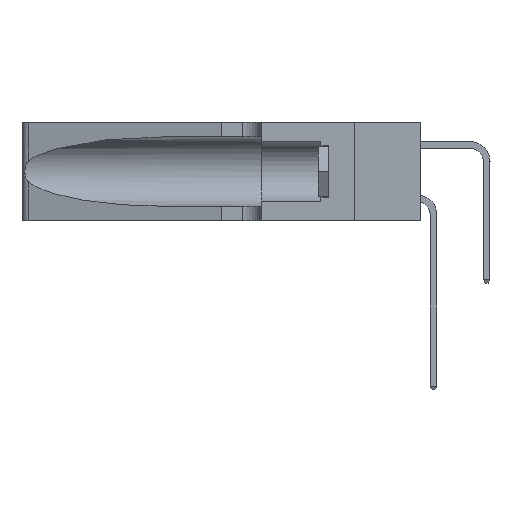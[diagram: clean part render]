
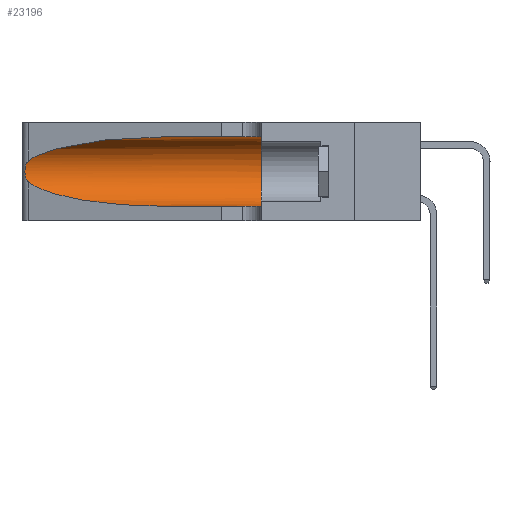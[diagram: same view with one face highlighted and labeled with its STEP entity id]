
A CAD part, left-side view. The second image highlights one B-rep face of the part: STEP entity #23196.
In plain terms, the highlighted cylindrical face has radius 3.308 mm (diameter 6.617 mm), a partial arc.
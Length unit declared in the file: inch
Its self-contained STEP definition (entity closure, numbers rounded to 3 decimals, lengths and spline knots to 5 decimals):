
#501 = CARTESIAN_POINT ( 'NONE',  ( 0.1305, 0.35, 0.31525 ) ) ;
#938 = CIRCLE ( 'NONE', #2635, 0.13025 ) ;
#1178 = AXIS2_PLACEMENT_3D ( 'NONE', #28094, #37419, #25106 ) ;
#1410 = CARTESIAN_POINT ( 'NONE',  ( 0.25487, 1.22718, 0.22369 ) ) ;
#1908 = CARTESIAN_POINT ( 'NONE',  ( 0.26018, 1.23835, 0.19895 ) ) ;
#2635 = AXIS2_PLACEMENT_3D ( 'NONE', #4890, #23425, #38960 ) ;
#3471 = CARTESIAN_POINT ( 'NONE',  ( 0.1305, 0.72297, 0.05475 ) ) ;
#3901 = VERTEX_POINT ( 'NONE', #39192 ) ;
#4736 = CARTESIAN_POINT ( 'NONE',  ( 0.25787, 1.23484, 0.2124 ) ) ;
#4890 = CARTESIAN_POINT ( 'NONE',  ( 0.1305, 0.35, 0.185 ) ) ;
#5528 = CARTESIAN_POINT ( 'NONE',  ( 0.25555, 1.22993, 0.14849 ) ) ;
#6198 = VERTEX_POINT ( 'NONE', #37043 ) ;
#7622 = CARTESIAN_POINT ( 'NONE',  ( 0.1305, 0.72297, 0.31525 ) ) ;
#8643 = ORIENTED_EDGE ( 'NONE', *, *, #38091, .T. ) ;
#9295 = CARTESIAN_POINT ( 'NONE',  ( 0.25487, 1.22718, 0.14631 ) ) ;
#9516 =( BOUNDED_CURVE ( )  B_SPLINE_CURVE ( 3, ( #13980, #20180, #32379, #16548 ),
 .UNSPECIFIED., .F., .T. ) 
 B_SPLINE_CURVE_WITH_KNOTS ( ( 4, 4 ),
 ( 1.5708, 2.84003 ),
 .UNSPECIFIED. ) 
 CURVE ( )  GEOMETRIC_REPRESENTATION_ITEM ( )  RATIONAL_B_SPLINE_CURVE ( ( 1., 0.87, 0.87, 1. ) ) 
 REPRESENTATION_ITEM ( '' )  );
#10037 = EDGE_CURVE ( 'NONE', #26850, #33340, #9516, .T. ) ;
#10630 = DIRECTION ( 'NONE',  ( 0., -1., 0. ) ) ;
#10841 = CARTESIAN_POINT ( 'NONE',  ( 0.25555, 1.22994, 0.2215 ) ) ;
#12903 = CYLINDRICAL_SURFACE ( 'NONE', #1178, 0.13025 ) ;
#13160 = LINE ( 'NONE', #38216, #28650 ) ;
#13615 = EDGE_CURVE ( 'NONE', #33340, #6198, #37051, .T. ) ;
#13980 = CARTESIAN_POINT ( 'NONE',  ( 0.1305, 0.72297, 0.31525 ) ) ;
#14177 = CARTESIAN_POINT ( 'NONE',  ( 0.25639, 1.23184, 0.21858 ) ) ;
#14317 = CARTESIAN_POINT ( 'NONE',  ( 0.26075, 1.23896, 0.19203 ) ) ;
#15771 = CARTESIAN_POINT ( 'NONE',  ( 0.18966, 0.96281, 0.05475 ) ) ;
#16548 = CARTESIAN_POINT ( 'NONE',  ( 0.25487, 1.22718, 0.22369 ) ) ;
#17108 = EDGE_CURVE ( 'NONE', #26850, #18586, #21584, .T. ) ;
#17307 = CARTESIAN_POINT ( 'NONE',  ( 0.26075, 1.23896, 0.178 ) ) ;
#17739 = ORIENTED_EDGE ( 'NONE', *, *, #13615, .T. ) ;
#18586 = VERTEX_POINT ( 'NONE', #501 ) ;
#18624 = CARTESIAN_POINT ( 'NONE',  ( 0.2373, 1.15595, 0.08982 ) ) ;
#19341 = ORIENTED_EDGE ( 'NONE', *, *, #17108, .F. ) ;
#20180 = CARTESIAN_POINT ( 'NONE',  ( 0.18966, 0.96281, 0.31525 ) ) ;
#20257 = CARTESIAN_POINT ( 'NONE',  ( 0.25487, 1.22718, 0.22369 ) ) ;
#21584 = LINE ( 'NONE', #36576, #24023 ) ;
#23081 = EDGE_LOOP ( 'NONE', ( #36023, #17739, #30147, #8643, #28327, #19341 ) ) ;
#23196 = ADVANCED_FACE ( 'NONE', ( #26982 ), #12903, .F. ) ;
#23425 = DIRECTION ( 'NONE',  ( 0., 1., 0. ) ) ;
#23883 = DIRECTION ( 'NONE',  ( 0., -1., 0. ) ) ;
#24023 = VECTOR ( 'NONE', #23883, 39.37008 ) ;
#25106 = DIRECTION ( 'NONE',  ( 0., 0., -1. ) ) ;
#26850 = VERTEX_POINT ( 'NONE', #7622 ) ;
#26982 = FACE_OUTER_BOUND ( 'NONE', #23081, .T. ) ;
#27190 = CARTESIAN_POINT ( 'NONE',  ( 0.25487, 1.22718, 0.14631 ) ) ;
#28094 = CARTESIAN_POINT ( 'NONE',  ( 0.1305, 1.61858, 0.185 ) ) ;
#28327 = ORIENTED_EDGE ( 'NONE', *, *, #32774, .F. ) ;
#28650 = VECTOR ( 'NONE', #10630, 39.37008 ) ;
#29889 = CARTESIAN_POINT ( 'NONE',  ( 0.25639, 1.23186, 0.15144 ) ) ;
#30147 = ORIENTED_EDGE ( 'NONE', *, *, #30730, .T. ) ;
#30158 = CARTESIAN_POINT ( 'NONE',  ( 0.25789, 1.23486, 0.15765 ) ) ;
#30730 = EDGE_CURVE ( 'NONE', #6198, #37258, #39515, .T. ) ;
#32379 = CARTESIAN_POINT ( 'NONE',  ( 0.2373, 1.15595, 0.28018 ) ) ;
#32774 = EDGE_CURVE ( 'NONE', #18586, #3901, #938, .T. ) ;
#32981 = CARTESIAN_POINT ( 'NONE',  ( 0.1305, 0.72297, 0.05475 ) ) ;
#33340 = VERTEX_POINT ( 'NONE', #1410 ) ;
#36023 = ORIENTED_EDGE ( 'NONE', *, *, #10037, .T. ) ;
#36576 = CARTESIAN_POINT ( 'NONE',  ( 0.1305, 1.61858, 0.31525 ) ) ;
#37043 = CARTESIAN_POINT ( 'NONE',  ( 0.25487, 1.22718, 0.14631 ) ) ;
#37051 = B_SPLINE_CURVE_WITH_KNOTS ( 'NONE', 3,
 ( #20257, #10841, #14177, #4736, #38285, #1908, #14317, #17307, #38931, #39195, #30158, #29889, #5528, #27190 ),
 .UNSPECIFIED., .F., .F.,
 ( 4, 2, 2, 2, 2, 2, 4 ),
 ( 0., 0.00027, 0.00053, 0.00107, 0.0016, 0.00187, 0.00214 ),
 .UNSPECIFIED. ) ;
#37258 = VERTEX_POINT ( 'NONE', #32981 ) ;
#37419 = DIRECTION ( 'NONE',  ( 0., -1., 0. ) ) ;
#38091 = EDGE_CURVE ( 'NONE', #37258, #3901, #13160, .T. ) ;
#38216 = CARTESIAN_POINT ( 'NONE',  ( 0.1305, 1.61858, 0.05475 ) ) ;
#38285 = CARTESIAN_POINT ( 'NONE',  ( 0.25854, 1.2359, 0.20912 ) ) ;
#38931 = CARTESIAN_POINT ( 'NONE',  ( 0.26017, 1.23833, 0.17102 ) ) ;
#38960 = DIRECTION ( 'NONE',  ( 0., 0., 1. ) ) ;
#39192 = CARTESIAN_POINT ( 'NONE',  ( 0.1305, 0.35, 0.05475 ) ) ;
#39195 = CARTESIAN_POINT ( 'NONE',  ( 0.25856, 1.23593, 0.16098 ) ) ;
#39515 =( BOUNDED_CURVE ( )  B_SPLINE_CURVE ( 3, ( #9295, #18624, #15771, #3471 ),
 .UNSPECIFIED., .F., .F. ) 
 B_SPLINE_CURVE_WITH_KNOTS ( ( 4, 4 ),
 ( 3.44316, 4.71239 ),
 .UNSPECIFIED. ) 
 CURVE ( )  GEOMETRIC_REPRESENTATION_ITEM ( )  RATIONAL_B_SPLINE_CURVE ( ( 1., 0.87, 0.87, 1. ) ) 
 REPRESENTATION_ITEM ( '' )  );
